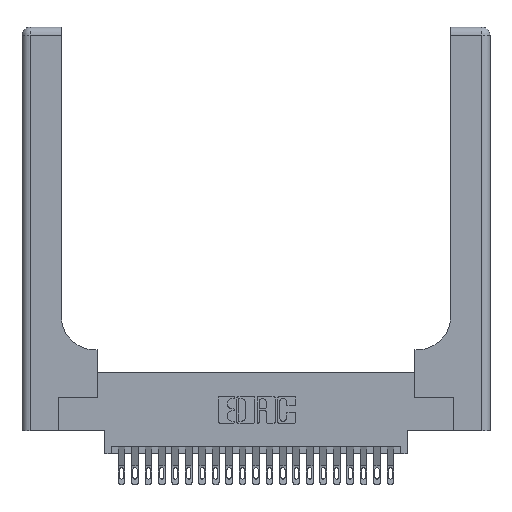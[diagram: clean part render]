
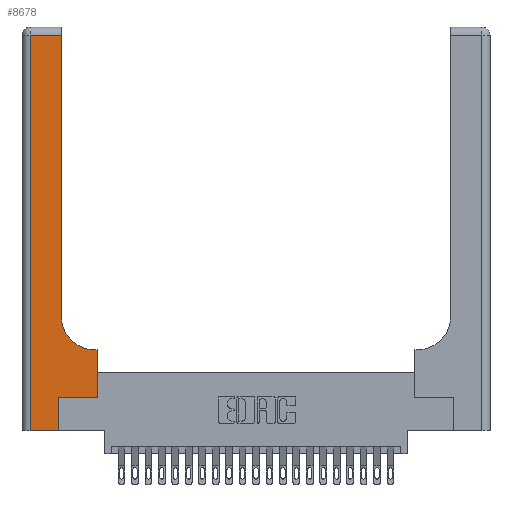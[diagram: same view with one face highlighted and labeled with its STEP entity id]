
A CAD part, top view. The second image highlights one B-rep face of the part: STEP entity #8678.
In plain terms, the highlighted planar face has unit normal (0, 0, 1).
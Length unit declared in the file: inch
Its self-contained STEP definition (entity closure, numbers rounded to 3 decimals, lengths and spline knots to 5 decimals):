
#248 = CARTESIAN_POINT ( 'NONE',  ( 0., 2.94, 0.37 ) ) ;
#333 = DIRECTION ( 'NONE',  ( -1., 0., 0. ) ) ;
#607 = VERTEX_POINT ( 'NONE', #7881 ) ;
#1286 = LINE ( 'NONE', #11645, #4312 ) ;
#1555 = EDGE_CURVE ( 'NONE', #11453, #24431, #6790, .T. ) ;
#2106 = CARTESIAN_POINT ( 'NONE',  ( 0., 3., 0.37 ) ) ;
#2149 = CARTESIAN_POINT ( 'NONE',  ( 0.2915, 2.94, 0.37 ) ) ;
#2429 = AXIS2_PLACEMENT_3D ( 'NONE', #5536, #14894, #3281 ) ;
#2884 = CARTESIAN_POINT ( 'NONE',  ( 0.06, 3., 0.37 ) ) ;
#3031 = EDGE_LOOP ( 'NONE', ( #18706, #3220, #22582, #7443, #10577, #11352, #8651, #3099, #12189 ) ) ;
#3099 = ORIENTED_EDGE ( 'NONE', *, *, #1555, .T. ) ;
#3191 = LINE ( 'NONE', #248, #11942 ) ;
#3220 = ORIENTED_EDGE ( 'NONE', *, *, #9364, .T. ) ;
#3281 = DIRECTION ( 'NONE',  ( 1., 0., 0. ) ) ;
#3411 = DIRECTION ( 'NONE',  ( 0., 1., 0. ) ) ;
#3701 = CARTESIAN_POINT ( 'NONE',  ( 0.06, 2.94, 0.37 ) ) ;
#4312 = VECTOR ( 'NONE', #5922, 39.37008 ) ;
#4367 = VERTEX_POINT ( 'NONE', #2149 ) ;
#4385 = CARTESIAN_POINT ( 'NONE',  ( 0.2915, 0.85, 0.37 ) ) ;
#4402 = CARTESIAN_POINT ( 'NONE',  ( 0.5585, 0.25, 0.37 ) ) ;
#4431 = CARTESIAN_POINT ( 'NONE',  ( 0., 0., 0.37 ) ) ;
#4682 = AXIS2_PLACEMENT_3D ( 'NONE', #2106, #17354, #9509 ) ;
#5104 = CARTESIAN_POINT ( 'NONE',  ( 0.5585, 0.25, 0.37 ) ) ;
#5320 = CARTESIAN_POINT ( 'NONE',  ( 0.2915, 0.6, 0.37 ) ) ;
#5489 = VECTOR ( 'NONE', #3411, 39.37008 ) ;
#5536 = CARTESIAN_POINT ( 'NONE',  ( 0.5415, 0.85, 0.37 ) ) ;
#5903 = PLANE ( 'NONE',  #4682 ) ;
#5922 = DIRECTION ( 'NONE',  ( 0., 1., 0. ) ) ;
#6790 = LINE ( 'NONE', #5320, #13722 ) ;
#7443 = ORIENTED_EDGE ( 'NONE', *, *, #18243, .T. ) ;
#7668 = VERTEX_POINT ( 'NONE', #24142 ) ;
#7881 = CARTESIAN_POINT ( 'NONE',  ( 0.06, 0., 0.37 ) ) ;
#8078 = EDGE_CURVE ( 'NONE', #17861, #11453, #9255, .T. ) ;
#8541 = VECTOR ( 'NONE', #19642, 39.37008 ) ;
#8651 = ORIENTED_EDGE ( 'NONE', *, *, #8078, .T. ) ;
#8678 = ADVANCED_FACE ( 'NONE', ( #16788 ), #5903, .F. ) ;
#8849 = CARTESIAN_POINT ( 'NONE',  ( 0.5415, 0.6, 0.37 ) ) ;
#9255 = LINE ( 'NONE', #4402, #16200 ) ;
#9364 = EDGE_CURVE ( 'NONE', #4367, #20835, #3191, .T. ) ;
#9509 = DIRECTION ( 'NONE',  ( -1., 0., 0. ) ) ;
#9676 = CARTESIAN_POINT ( 'NONE',  ( 0.269, 0.25, 0.37 ) ) ;
#10577 = ORIENTED_EDGE ( 'NONE', *, *, #16609, .T. ) ;
#11352 = ORIENTED_EDGE ( 'NONE', *, *, #19581, .T. ) ;
#11453 = VERTEX_POINT ( 'NONE', #16420 ) ;
#11645 = CARTESIAN_POINT ( 'NONE',  ( 0.2915, 3., 0.37 ) ) ;
#11942 = VECTOR ( 'NONE', #333, 39.37008 ) ;
#12189 = ORIENTED_EDGE ( 'NONE', *, *, #18003, .T. ) ;
#12985 = LINE ( 'NONE', #2884, #14494 ) ;
#13686 = VECTOR ( 'NONE', #13950, 39.37008 ) ;
#13722 = VECTOR ( 'NONE', #24798, 39.37008 ) ;
#13950 = DIRECTION ( 'NONE',  ( 1., 0., 0. ) ) ;
#14395 = CARTESIAN_POINT ( 'NONE',  ( 0.269, 0., 0.37 ) ) ;
#14494 = VECTOR ( 'NONE', #23861, 39.37008 ) ;
#14894 = DIRECTION ( 'NONE',  ( 0., 0., -1. ) ) ;
#16200 = VECTOR ( 'NONE', #17554, 39.37008 ) ;
#16285 = EDGE_CURVE ( 'NONE', #23140, #4367, #1286, .T. ) ;
#16420 = CARTESIAN_POINT ( 'NONE',  ( 0.5585, 0.6, 0.37 ) ) ;
#16609 = EDGE_CURVE ( 'NONE', #19617, #7668, #18476, .T. ) ;
#16719 = LINE ( 'NONE', #4431, #13686 ) ;
#16788 = FACE_OUTER_BOUND ( 'NONE', #3031, .T. ) ;
#17354 = DIRECTION ( 'NONE',  ( 0., 0., -1. ) ) ;
#17554 = DIRECTION ( 'NONE',  ( 0., 1., 0. ) ) ;
#17861 = VERTEX_POINT ( 'NONE', #5104 ) ;
#18003 = EDGE_CURVE ( 'NONE', #24431, #23140, #23072, .T. ) ;
#18243 = EDGE_CURVE ( 'NONE', #607, #19617, #16719, .T. ) ;
#18476 = LINE ( 'NONE', #22623, #5489 ) ;
#18706 = ORIENTED_EDGE ( 'NONE', *, *, #16285, .T. ) ;
#19581 = EDGE_CURVE ( 'NONE', #7668, #17861, #23045, .T. ) ;
#19617 = VERTEX_POINT ( 'NONE', #14395 ) ;
#19642 = DIRECTION ( 'NONE',  ( 1., 0., 0. ) ) ;
#20835 = VERTEX_POINT ( 'NONE', #3701 ) ;
#22582 = ORIENTED_EDGE ( 'NONE', *, *, #24789, .T. ) ;
#22623 = CARTESIAN_POINT ( 'NONE',  ( 0.269, 0., 0.37 ) ) ;
#23045 = LINE ( 'NONE', #9676, #8541 ) ;
#23072 = CIRCLE ( 'NONE', #2429, 0.25 ) ;
#23140 = VERTEX_POINT ( 'NONE', #4385 ) ;
#23861 = DIRECTION ( 'NONE',  ( 0., -1., 0. ) ) ;
#24142 = CARTESIAN_POINT ( 'NONE',  ( 0.269, 0.25, 0.37 ) ) ;
#24431 = VERTEX_POINT ( 'NONE', #8849 ) ;
#24789 = EDGE_CURVE ( 'NONE', #20835, #607, #12985, .T. ) ;
#24798 = DIRECTION ( 'NONE',  ( -1., 0., 0. ) ) ;
